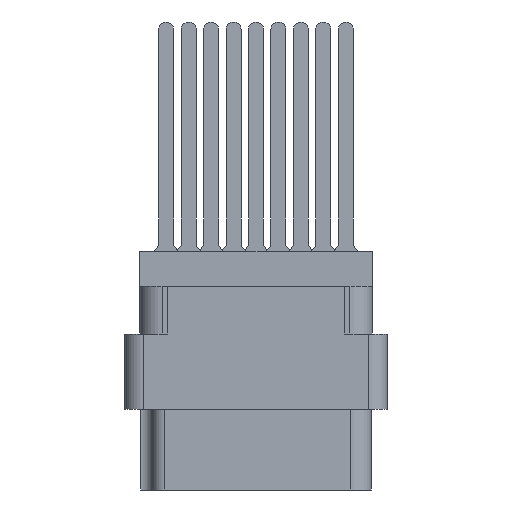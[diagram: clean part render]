
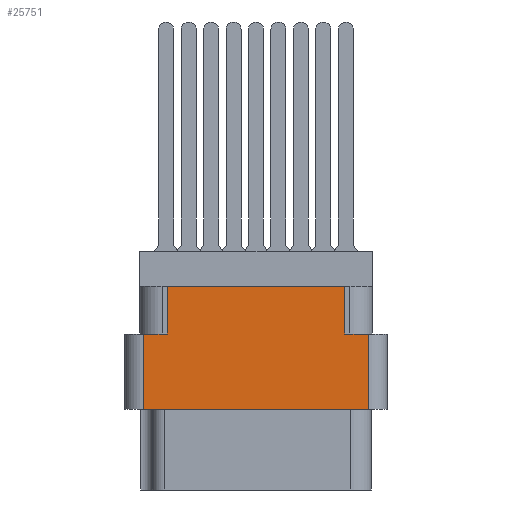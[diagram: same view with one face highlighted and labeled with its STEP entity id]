
A CAD part, left-side view. The second image highlights one B-rep face of the part: STEP entity #25751.
In plain terms, the highlighted planar face has unit normal (-1, 0, 0).
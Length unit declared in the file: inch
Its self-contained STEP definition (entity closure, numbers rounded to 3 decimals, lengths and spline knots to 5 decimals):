
#425 = CARTESIAN_POINT ( 'NONE',  ( -1.296, 0., -0.277 ) ) ;
#447 = VERTEX_POINT ( 'NONE', #39867 ) ;
#2572 = DIRECTION ( 'NONE',  ( 0., 0., -1. ) ) ;
#2903 = VECTOR ( 'NONE', #23691, 39.37008 ) ;
#3273 = CARTESIAN_POINT ( 'NONE',  ( -1.296, 0.376, -0.277 ) ) ;
#3299 = CARTESIAN_POINT ( 'NONE',  ( -1.296, 0., -0.277 ) ) ;
#3374 = VECTOR ( 'NONE', #32670, 39.37008 ) ;
#4654 = VECTOR ( 'NONE', #42731, 39.37008 ) ;
#5254 = CARTESIAN_POINT ( 'NONE',  ( -1.296, 0.296, -0.117 ) ) ;
#5810 = ORIENTED_EDGE ( 'NONE', *, *, #21223, .T. ) ;
#6283 = ORIENTED_EDGE ( 'NONE', *, *, #18834, .F. ) ;
#7255 = VERTEX_POINT ( 'NONE', #3273 ) ;
#7475 = DIRECTION ( 'NONE',  ( 0., 0., 1. ) ) ;
#8097 = VERTEX_POINT ( 'NONE', #38249 ) ;
#8903 = PLANE ( 'NONE',  #44399 ) ;
#9490 = VECTOR ( 'NONE', #2572, 39.37008 ) ;
#10872 = ORIENTED_EDGE ( 'NONE', *, *, #42523, .F. ) ;
#14580 = VECTOR ( 'NONE', #28178, 39.37008 ) ;
#15275 = LINE ( 'NONE', #51071, #34431 ) ;
#15304 = ORIENTED_EDGE ( 'NONE', *, *, #20616, .F. ) ;
#15873 = EDGE_LOOP ( 'NONE', ( #6283, #5810, #10872, #32360, #15304, #38081, #17632, #44763 ) ) ;
#16799 = CARTESIAN_POINT ( 'NONE',  ( -1.296, -0.438, -0.798 ) ) ;
#17463 = LINE ( 'NONE', #26191, #9490 ) ;
#17632 = ORIENTED_EDGE ( 'NONE', *, *, #38640, .F. ) ;
#18683 = CARTESIAN_POINT ( 'NONE',  ( -1.296, 0.296, -0.277 ) ) ;
#18834 = EDGE_CURVE ( 'NONE', #7255, #23840, #23873, .T. ) ;
#19245 = VERTEX_POINT ( 'NONE', #26373 ) ;
#19441 = VECTOR ( 'NONE', #43349, 39.37008 ) ;
#20246 = DIRECTION ( 'NONE',  ( -1., 0., 0. ) ) ;
#20616 = EDGE_CURVE ( 'NONE', #447, #29968, #22536, .T. ) ;
#21223 = EDGE_CURVE ( 'NONE', #7255, #19245, #17463, .T. ) ;
#22536 = LINE ( 'NONE', #3299, #19441 ) ;
#23691 = DIRECTION ( 'NONE',  ( 0., -1., 0. ) ) ;
#23840 = VERTEX_POINT ( 'NONE', #28059 ) ;
#23873 = LINE ( 'NONE', #425, #2903 ) ;
#24567 = FACE_OUTER_BOUND ( 'NONE', #15873, .T. ) ;
#25224 = CARTESIAN_POINT ( 'NONE',  ( -1.296, 0.438, -0.117 ) ) ;
#25751 = ADVANCED_FACE ( 'NONE', ( #24567 ), #8903, .T. ) ;
#26191 = CARTESIAN_POINT ( 'NONE',  ( -1.296, 0.376, -0.798 ) ) ;
#26373 = CARTESIAN_POINT ( 'NONE',  ( -1.296, 0.376, -0.529 ) ) ;
#27148 = CARTESIAN_POINT ( 'NONE',  ( -1.296, -0.296, -0.277 ) ) ;
#27717 = DIRECTION ( 'NONE',  ( 0., 1., 0. ) ) ;
#28059 = CARTESIAN_POINT ( 'NONE',  ( -1.296, 0.296, -0.277 ) ) ;
#28178 = DIRECTION ( 'NONE',  ( 0., 0., 1. ) ) ;
#28513 = CARTESIAN_POINT ( 'NONE',  ( -1.296, -0.376, -0.529 ) ) ;
#28755 = DIRECTION ( 'NONE',  ( 0., 0., 1. ) ) ;
#29137 = VERTEX_POINT ( 'NONE', #28513 ) ;
#29968 = VERTEX_POINT ( 'NONE', #41363 ) ;
#30673 = LINE ( 'NONE', #27148, #43681 ) ;
#32360 = ORIENTED_EDGE ( 'NONE', *, *, #43229, .T. ) ;
#32670 = DIRECTION ( 'NONE',  ( 0., -1., 0. ) ) ;
#32681 = VERTEX_POINT ( 'NONE', #5254 ) ;
#34431 = VECTOR ( 'NONE', #27717, 39.37008 ) ;
#34869 = LINE ( 'NONE', #25224, #3374 ) ;
#38081 = ORIENTED_EDGE ( 'NONE', *, *, #43075, .T. ) ;
#38192 = EDGE_CURVE ( 'NONE', #23840, #32681, #44187, .T. ) ;
#38249 = CARTESIAN_POINT ( 'NONE',  ( -1.296, -0.296, -0.117 ) ) ;
#38640 = EDGE_CURVE ( 'NONE', #32681, #8097, #34869, .T. ) ;
#39234 = CARTESIAN_POINT ( 'NONE',  ( -1.296, -0.376, -0.798 ) ) ;
#39867 = CARTESIAN_POINT ( 'NONE',  ( -1.296, -0.296, -0.277 ) ) ;
#41363 = CARTESIAN_POINT ( 'NONE',  ( -1.296, -0.376, -0.277 ) ) ;
#41787 = LINE ( 'NONE', #39234, #14580 ) ;
#42523 = EDGE_CURVE ( 'NONE', #29137, #19245, #15275, .T. ) ;
#42731 = DIRECTION ( 'NONE',  ( 0., 0., 1. ) ) ;
#43075 = EDGE_CURVE ( 'NONE', #447, #8097, #30673, .T. ) ;
#43229 = EDGE_CURVE ( 'NONE', #29137, #29968, #41787, .T. ) ;
#43349 = DIRECTION ( 'NONE',  ( 0., -1., 0. ) ) ;
#43681 = VECTOR ( 'NONE', #7475, 39.37008 ) ;
#44187 = LINE ( 'NONE', #18683, #4654 ) ;
#44399 = AXIS2_PLACEMENT_3D ( 'NONE', #16799, #20246, #28755 ) ;
#44763 = ORIENTED_EDGE ( 'NONE', *, *, #38192, .F. ) ;
#51071 = CARTESIAN_POINT ( 'NONE',  ( -1.296, 0., -0.529 ) ) ;
